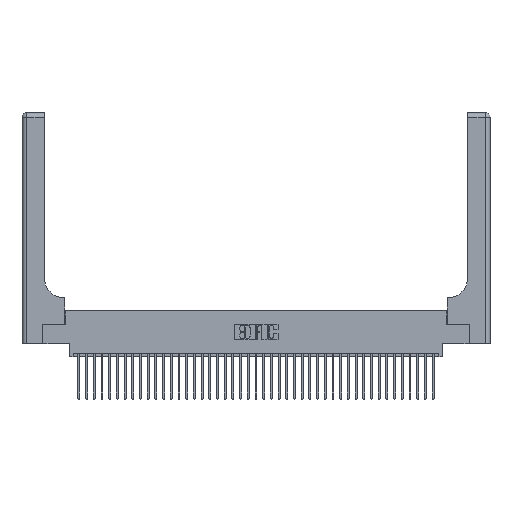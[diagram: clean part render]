
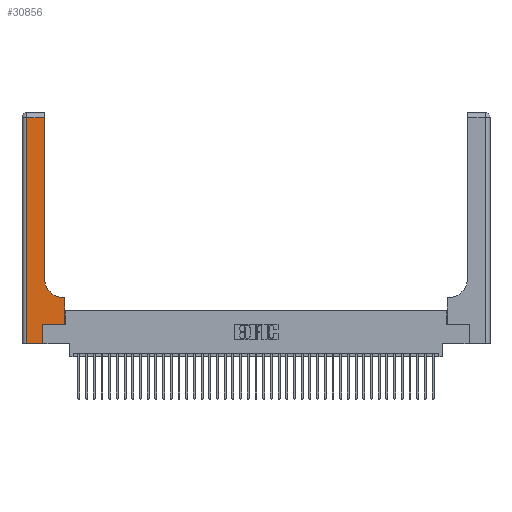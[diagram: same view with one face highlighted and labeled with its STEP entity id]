
A CAD part, top view. The second image highlights one B-rep face of the part: STEP entity #30856.
In plain terms, the highlighted planar face has unit normal (0, 0, 1).
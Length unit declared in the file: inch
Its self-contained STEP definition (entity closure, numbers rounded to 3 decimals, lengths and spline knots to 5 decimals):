
#296 = ORIENTED_EDGE ( 'NONE', *, *, #36778, .T. ) ;
#330 = VERTEX_POINT ( 'NONE', #35560 ) ;
#883 = AXIS2_PLACEMENT_3D ( 'NONE', #7615, #10844, #39897 ) ;
#1087 = VECTOR ( 'NONE', #28473, 39.37008 ) ;
#1698 = ORIENTED_EDGE ( 'NONE', *, *, #34836, .T. ) ;
#2555 = ORIENTED_EDGE ( 'NONE', *, *, #21815, .T. ) ;
#2761 = CARTESIAN_POINT ( 'NONE',  ( 0., 2.94, 0.37 ) ) ;
#3531 = EDGE_CURVE ( 'NONE', #17746, #8703, #20087, .T. ) ;
#3723 = LINE ( 'NONE', #17161, #25347 ) ;
#4286 = CARTESIAN_POINT ( 'NONE',  ( 0.2915, 2.94, 0.37 ) ) ;
#4765 = LINE ( 'NONE', #12575, #12310 ) ;
#5614 = EDGE_CURVE ( 'NONE', #8651, #5838, #30046, .T. ) ;
#5699 = CARTESIAN_POINT ( 'NONE',  ( 0.5585, 0.6, 0.37 ) ) ;
#5838 = VERTEX_POINT ( 'NONE', #21368 ) ;
#6684 = DIRECTION ( 'NONE',  ( 1., 0., 0. ) ) ;
#6789 = ORIENTED_EDGE ( 'NONE', *, *, #33755, .T. ) ;
#6839 = VECTOR ( 'NONE', #35064, 39.37008 ) ;
#7615 = CARTESIAN_POINT ( 'NONE',  ( 0., 3., 0.37 ) ) ;
#8651 = VERTEX_POINT ( 'NONE', #36734 ) ;
#8703 = VERTEX_POINT ( 'NONE', #5699 ) ;
#9083 = DIRECTION ( 'NONE',  ( 0., -1., 0. ) ) ;
#9457 = LINE ( 'NONE', #10200, #30507 ) ;
#10200 = CARTESIAN_POINT ( 'NONE',  ( 0.269, 0.25, 0.37 ) ) ;
#10844 = DIRECTION ( 'NONE',  ( 0., 0., -1. ) ) ;
#12310 = VECTOR ( 'NONE', #9083, 39.37008 ) ;
#12575 = CARTESIAN_POINT ( 'NONE',  ( 0.06, 3., 0.37 ) ) ;
#12762 = EDGE_CURVE ( 'NONE', #16801, #16224, #35352, .T. ) ;
#13013 = DIRECTION ( 'NONE',  ( 0., 0., -1. ) ) ;
#14090 = CARTESIAN_POINT ( 'NONE',  ( 0.06, 0., 0.37 ) ) ;
#14182 = CARTESIAN_POINT ( 'NONE',  ( 0.06, 2.94, 0.37 ) ) ;
#15119 = VECTOR ( 'NONE', #15214, 39.37008 ) ;
#15214 = DIRECTION ( 'NONE',  ( 0., 1., 0. ) ) ;
#15492 = ORIENTED_EDGE ( 'NONE', *, *, #12762, .T. ) ;
#15564 = CARTESIAN_POINT ( 'NONE',  ( 0.5585, 0.25, 0.37 ) ) ;
#16224 = VERTEX_POINT ( 'NONE', #14182 ) ;
#16801 = VERTEX_POINT ( 'NONE', #4286 ) ;
#17161 = CARTESIAN_POINT ( 'NONE',  ( 0.2915, 0.6, 0.37 ) ) ;
#17746 = VERTEX_POINT ( 'NONE', #15564 ) ;
#18398 = LINE ( 'NONE', #32109, #6839 ) ;
#18688 = EDGE_CURVE ( 'NONE', #5838, #17746, #9457, .T. ) ;
#18738 = AXIS2_PLACEMENT_3D ( 'NONE', #19480, #13013, #6684 ) ;
#19371 = FACE_OUTER_BOUND ( 'NONE', #28333, .T. ) ;
#19480 = CARTESIAN_POINT ( 'NONE',  ( 0.5415, 0.85, 0.37 ) ) ;
#20087 = LINE ( 'NONE', #25337, #15119 ) ;
#20388 = EDGE_CURVE ( 'NONE', #16224, #39116, #4765, .T. ) ;
#20762 = VERTEX_POINT ( 'NONE', #32768 ) ;
#21368 = CARTESIAN_POINT ( 'NONE',  ( 0.269, 0.25, 0.37 ) ) ;
#21815 = EDGE_CURVE ( 'NONE', #8703, #20762, #3723, .T. ) ;
#22043 = DIRECTION ( 'NONE',  ( 0., 1., 0. ) ) ;
#25178 = ORIENTED_EDGE ( 'NONE', *, *, #5614, .T. ) ;
#25337 = CARTESIAN_POINT ( 'NONE',  ( 0.5585, 0.25, 0.37 ) ) ;
#25347 = VECTOR ( 'NONE', #39870, 39.37008 ) ;
#28333 = EDGE_LOOP ( 'NONE', ( #296, #15492, #38948, #6789, #25178, #28664, #33991, #2555, #1698 ) ) ;
#28473 = DIRECTION ( 'NONE',  ( 1., 0., 0. ) ) ;
#28657 = CIRCLE ( 'NONE', #18738, 0.25 ) ;
#28664 = ORIENTED_EDGE ( 'NONE', *, *, #18688, .T. ) ;
#30046 = LINE ( 'NONE', #31572, #38097 ) ;
#30507 = VECTOR ( 'NONE', #32932, 39.37008 ) ;
#30856 = ADVANCED_FACE ( 'NONE', ( #19371 ), #33319, .F. ) ;
#31572 = CARTESIAN_POINT ( 'NONE',  ( 0.269, 0., 0.37 ) ) ;
#32109 = CARTESIAN_POINT ( 'NONE',  ( 0.2915, 3., 0.37 ) ) ;
#32755 = LINE ( 'NONE', #38536, #1087 ) ;
#32768 = CARTESIAN_POINT ( 'NONE',  ( 0.5415, 0.6, 0.37 ) ) ;
#32932 = DIRECTION ( 'NONE',  ( 1., 0., 0. ) ) ;
#33319 = PLANE ( 'NONE',  #883 ) ;
#33330 = VECTOR ( 'NONE', #34588, 39.37008 ) ;
#33755 = EDGE_CURVE ( 'NONE', #39116, #8651, #32755, .T. ) ;
#33991 = ORIENTED_EDGE ( 'NONE', *, *, #3531, .T. ) ;
#34588 = DIRECTION ( 'NONE',  ( -1., 0., 0. ) ) ;
#34836 = EDGE_CURVE ( 'NONE', #20762, #330, #28657, .T. ) ;
#35064 = DIRECTION ( 'NONE',  ( 0., 1., 0. ) ) ;
#35352 = LINE ( 'NONE', #2761, #33330 ) ;
#35560 = CARTESIAN_POINT ( 'NONE',  ( 0.2915, 0.85, 0.37 ) ) ;
#36734 = CARTESIAN_POINT ( 'NONE',  ( 0.269, 0., 0.37 ) ) ;
#36778 = EDGE_CURVE ( 'NONE', #330, #16801, #18398, .T. ) ;
#38097 = VECTOR ( 'NONE', #22043, 39.37008 ) ;
#38536 = CARTESIAN_POINT ( 'NONE',  ( 0., 0., 0.37 ) ) ;
#38948 = ORIENTED_EDGE ( 'NONE', *, *, #20388, .T. ) ;
#39116 = VERTEX_POINT ( 'NONE', #14090 ) ;
#39870 = DIRECTION ( 'NONE',  ( -1., 0., 0. ) ) ;
#39897 = DIRECTION ( 'NONE',  ( -1., 0., 0. ) ) ;
